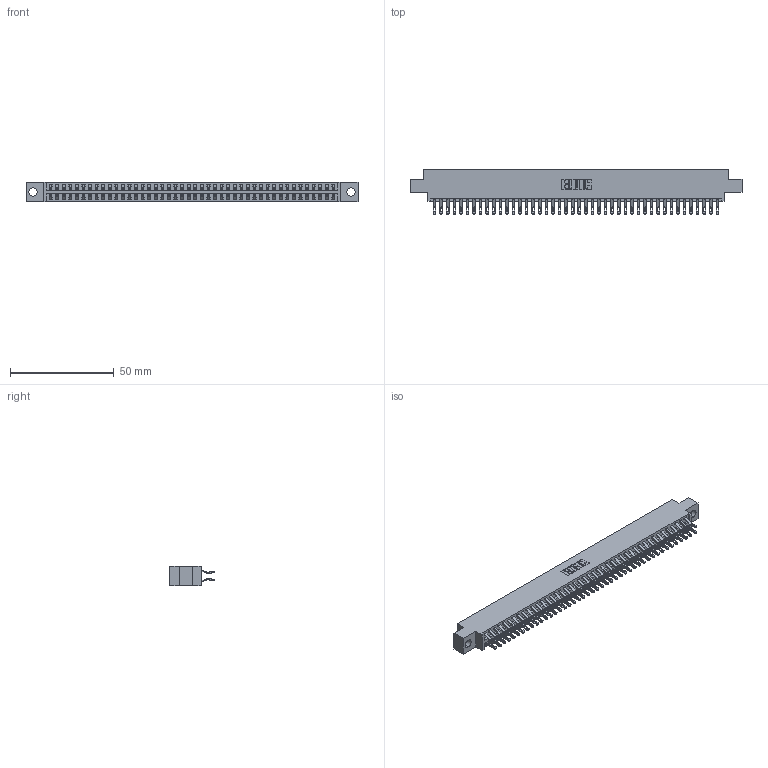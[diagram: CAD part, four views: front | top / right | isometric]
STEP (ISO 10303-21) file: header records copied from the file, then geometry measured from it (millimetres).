
FILE_DESCRIPTION (( 'STEP AP203' ), '1' );
FILE_NAME ('396-088-555-804.STEP', '2019-11-02T15:14:17', ( '' ), ( '' ), 'SwSTEP 2.0', 'SolidWorks 2016', '' );
FILE_SCHEMA (( 'CONFIG_CONTROL_DESIGN' ));
Length unit declared in the file: inch
Products named in the file (3): 396-088-555-804; 346 Part_0.170 Offset - 0.156 Dia-TH; 345-292-001_555 Tail
Assembly tree (89 placements, depth 2):
  396-088-555-804
    346 Part_0.170 Offset - 0.156 Dia-TH
    345-292-001_555 Tail  x88
Bounding box: 160.27 x 21.46 x 9.4 mm (x, y, z)
Volume: 15657 mm3; surface area: 22455.9 mm2
Topology: 89 solids, 89 shells, 5230 faces, 16445 edges, 10962 vertices
Faces by surface type: plane 2984, cylinder 2246
Entity records: 28907 total; most frequent: CARTESIAN_POINT 4798, ORIENTED_EDGE 4702, DIRECTION 4247, EDGE_CURVE 2351, VECTOR 2023, LINE 2023, VERTEX_POINT 1566, AXIS2_PLACEMENT_3D 1112
